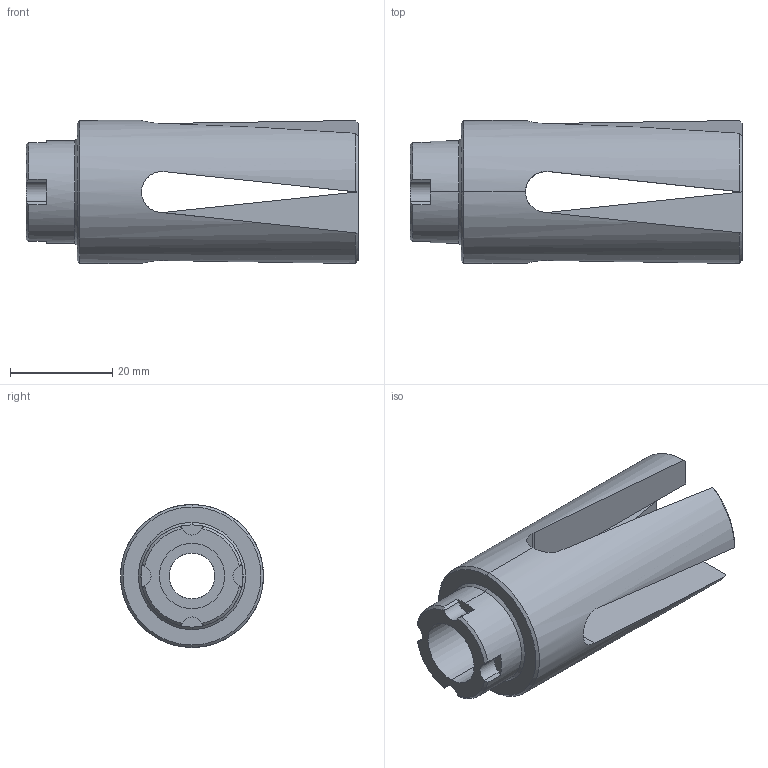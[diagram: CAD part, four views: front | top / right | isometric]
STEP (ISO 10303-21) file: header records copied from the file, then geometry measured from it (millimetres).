
FILE_DESCRIPTION (( 'STEP AP214' ), '1' );
FILE_NAME ('Flashhider_vortex.STEP', '2013-06-19T08:24:15', ( 'fireraisr' ), ( '' ), 'SwSTEP 2.0', 'SolidWorks 2012', '' );
FILE_SCHEMA (( 'AUTOMOTIVE_DESIGN' ));
Length unit declared in the file: millimetre
Products named in the file (1): Flashhider_vortex
Bounding box: 65 x 28 x 28 mm (x, y, z)
Volume: 18161.3 mm3; surface area: 8972.1 mm2
Topology: 1 solids, 1 shells, 64 faces, 176 edges, 116 vertices
Faces by surface type: plane 28, cylinder 23, cone 13
Entity records: 2320 total; most frequent: CARTESIAN_POINT 736, ORIENTED_EDGE 352, DIRECTION 288, EDGE_CURVE 176, VERTEX_POINT 116, AXIS2_PLACEMENT_3D 116, EDGE_LOOP 68, ADVANCED_FACE 64
